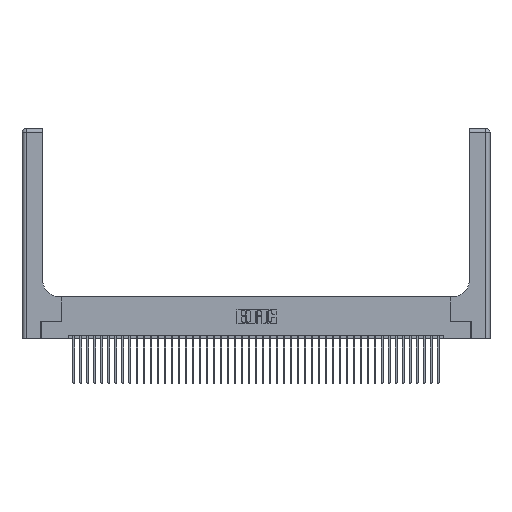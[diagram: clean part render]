
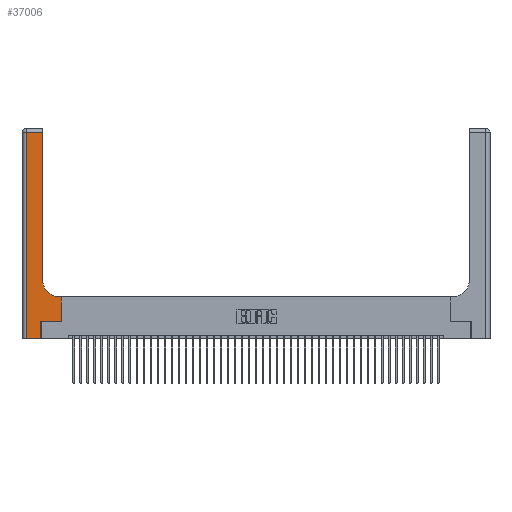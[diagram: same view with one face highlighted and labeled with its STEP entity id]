
A CAD part, top view. The second image highlights one B-rep face of the part: STEP entity #37006.
In plain terms, the highlighted planar face has unit normal (0, 0, 1).
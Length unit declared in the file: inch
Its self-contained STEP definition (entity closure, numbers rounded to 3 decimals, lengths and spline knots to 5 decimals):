
#628 = ORIENTED_EDGE ( 'NONE', *, *, #31290, .T. ) ;
#1177 = EDGE_LOOP ( 'NONE', ( #2159, #11992, #14433, #5083, #44691, #28079, #38960, #628, #18469 ) ) ;
#1439 = DIRECTION ( 'NONE',  ( 0., 1., 0. ) ) ;
#1865 = CARTESIAN_POINT ( 'NONE',  ( 0.2915, 2.94, 0.37 ) ) ;
#2159 = ORIENTED_EDGE ( 'NONE', *, *, #42554, .T. ) ;
#2314 = DIRECTION ( 'NONE',  ( -1., 0., 0. ) ) ;
#2502 = VECTOR ( 'NONE', #25155, 39.37008 ) ;
#2910 = LINE ( 'NONE', #23119, #30368 ) ;
#2970 = CARTESIAN_POINT ( 'NONE',  ( 0.269, 0.25, 0.37 ) ) ;
#3459 = DIRECTION ( 'NONE',  ( -1., 0., 0. ) ) ;
#3844 = VERTEX_POINT ( 'NONE', #10210 ) ;
#4937 = CARTESIAN_POINT ( 'NONE',  ( 0.5415, 0.85, 0.37 ) ) ;
#5083 = ORIENTED_EDGE ( 'NONE', *, *, #33472, .T. ) ;
#5480 = DIRECTION ( 'NONE',  ( 0., 1., 0. ) ) ;
#7726 = VERTEX_POINT ( 'NONE', #13584 ) ;
#8166 = DIRECTION ( 'NONE',  ( 1., 0., 0. ) ) ;
#9231 = AXIS2_PLACEMENT_3D ( 'NONE', #4937, #29135, #8166 ) ;
#9882 = VERTEX_POINT ( 'NONE', #11784 ) ;
#10210 = CARTESIAN_POINT ( 'NONE',  ( 0.269, 0.25, 0.37 ) ) ;
#10498 = LINE ( 'NONE', #2970, #31327 ) ;
#11222 = CIRCLE ( 'NONE', #9231, 0.25 ) ;
#11784 = CARTESIAN_POINT ( 'NONE',  ( 0.06, 0., 0.37 ) ) ;
#11850 = LINE ( 'NONE', #42611, #2502 ) ;
#11872 = CARTESIAN_POINT ( 'NONE',  ( 0.269, 0., 0.37 ) ) ;
#11992 = ORIENTED_EDGE ( 'NONE', *, *, #15188, .T. ) ;
#13093 = LINE ( 'NONE', #36688, #30036 ) ;
#13154 = CARTESIAN_POINT ( 'NONE',  ( 0.5585, 0.6, 0.37 ) ) ;
#13584 = CARTESIAN_POINT ( 'NONE',  ( 0.5415, 0.6, 0.37 ) ) ;
#14433 = ORIENTED_EDGE ( 'NONE', *, *, #14982, .T. ) ;
#14982 = EDGE_CURVE ( 'NONE', #20624, #9882, #43651, .T. ) ;
#15188 = EDGE_CURVE ( 'NONE', #31814, #20624, #20102, .T. ) ;
#16150 = CARTESIAN_POINT ( 'NONE',  ( 0.5585, 0.25, 0.37 ) ) ;
#17598 = DIRECTION ( 'NONE',  ( 0., -1., 0. ) ) ;
#17844 = VECTOR ( 'NONE', #1439, 39.37008 ) ;
#18469 = ORIENTED_EDGE ( 'NONE', *, *, #22823, .T. ) ;
#20102 = LINE ( 'NONE', #35291, #39180 ) ;
#20624 = VERTEX_POINT ( 'NONE', #23112 ) ;
#21642 = LINE ( 'NONE', #29690, #17844 ) ;
#22279 = CARTESIAN_POINT ( 'NONE',  ( 0.269, 0., 0.37 ) ) ;
#22823 = EDGE_CURVE ( 'NONE', #7726, #43961, #11222, .T. ) ;
#23112 = CARTESIAN_POINT ( 'NONE',  ( 0.06, 2.94, 0.37 ) ) ;
#23119 = CARTESIAN_POINT ( 'NONE',  ( 0.2915, 0.6, 0.37 ) ) ;
#23341 = CARTESIAN_POINT ( 'NONE',  ( 0., 3., 0.37 ) ) ;
#23563 = CARTESIAN_POINT ( 'NONE',  ( 0.2915, 0.85, 0.37 ) ) ;
#24927 = EDGE_CURVE ( 'NONE', #3844, #30166, #10498, .T. ) ;
#25155 = DIRECTION ( 'NONE',  ( 1., 0., 0. ) ) ;
#26464 = DIRECTION ( 'NONE',  ( -1., 0., 0. ) ) ;
#28079 = ORIENTED_EDGE ( 'NONE', *, *, #24927, .T. ) ;
#29135 = DIRECTION ( 'NONE',  ( 0., 0., -1. ) ) ;
#29190 = AXIS2_PLACEMENT_3D ( 'NONE', #23341, #30094, #2314 ) ;
#29690 = CARTESIAN_POINT ( 'NONE',  ( 0.5585, 0.25, 0.37 ) ) ;
#30036 = VECTOR ( 'NONE', #5480, 39.37008 ) ;
#30094 = DIRECTION ( 'NONE',  ( 0., 0., -1. ) ) ;
#30166 = VERTEX_POINT ( 'NONE', #16150 ) ;
#30368 = VECTOR ( 'NONE', #26464, 39.37008 ) ;
#31290 = EDGE_CURVE ( 'NONE', #34443, #7726, #2910, .T. ) ;
#31327 = VECTOR ( 'NONE', #34660, 39.37008 ) ;
#31814 = VERTEX_POINT ( 'NONE', #1865 ) ;
#33207 = VECTOR ( 'NONE', #17598, 39.37008 ) ;
#33395 = LINE ( 'NONE', #11872, #40018 ) ;
#33472 = EDGE_CURVE ( 'NONE', #9882, #43148, #11850, .T. ) ;
#34101 = EDGE_CURVE ( 'NONE', #30166, #34443, #21642, .T. ) ;
#34443 = VERTEX_POINT ( 'NONE', #13154 ) ;
#34660 = DIRECTION ( 'NONE',  ( 1., 0., 0. ) ) ;
#35291 = CARTESIAN_POINT ( 'NONE',  ( 0., 2.94, 0.37 ) ) ;
#36688 = CARTESIAN_POINT ( 'NONE',  ( 0.2915, 3., 0.37 ) ) ;
#37006 = ADVANCED_FACE ( 'NONE', ( #42740 ), #44283, .F. ) ;
#38960 = ORIENTED_EDGE ( 'NONE', *, *, #34101, .T. ) ;
#39180 = VECTOR ( 'NONE', #3459, 39.37008 ) ;
#40018 = VECTOR ( 'NONE', #40182, 39.37008 ) ;
#40182 = DIRECTION ( 'NONE',  ( 0., 1., 0. ) ) ;
#41287 = EDGE_CURVE ( 'NONE', #43148, #3844, #33395, .T. ) ;
#41435 = CARTESIAN_POINT ( 'NONE',  ( 0.06, 3., 0.37 ) ) ;
#42554 = EDGE_CURVE ( 'NONE', #43961, #31814, #13093, .T. ) ;
#42611 = CARTESIAN_POINT ( 'NONE',  ( 0., 0., 0.37 ) ) ;
#42740 = FACE_OUTER_BOUND ( 'NONE', #1177, .T. ) ;
#43148 = VERTEX_POINT ( 'NONE', #22279 ) ;
#43651 = LINE ( 'NONE', #41435, #33207 ) ;
#43961 = VERTEX_POINT ( 'NONE', #23563 ) ;
#44283 = PLANE ( 'NONE',  #29190 ) ;
#44691 = ORIENTED_EDGE ( 'NONE', *, *, #41287, .T. ) ;
